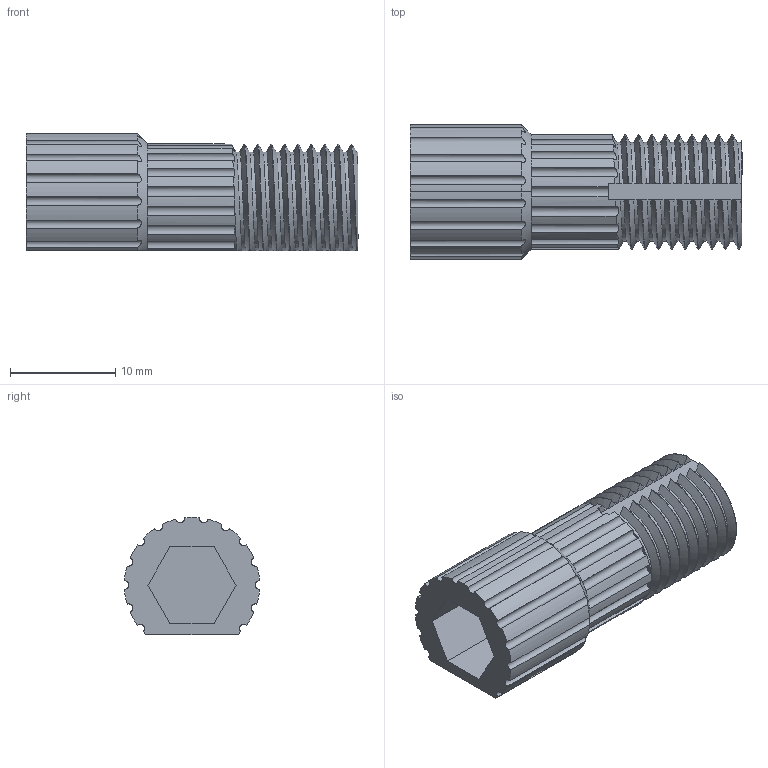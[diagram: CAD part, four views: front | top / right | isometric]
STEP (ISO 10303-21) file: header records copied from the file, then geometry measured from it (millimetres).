
FILE_DESCRIPTION (( 'STEP AP203' ), '1' );
FILE_NAME ('AF-HF-LR-PRT-003-STEP.STEP', '2020-10-04T16:07:10', ( '' ), ( '' ), 'SwSTEP 2.0', 'SolidWorks 2018', '' );
FILE_SCHEMA (( 'CONFIG_CONTROL_DESIGN' ));
Products named in the file (1): AF-HF-LR-PRT-003-STEP
Bounding box: 31.5 x 12.81 x 11.12 mm (x, y, z)
Volume: 2442.1 mm3; surface area: 1936.2 mm2
Topology: 1 solids, 1 shells, 232 faces, 599 edges, 371 vertices
Faces by surface type: cylinder 90, plane 81, bspline 59, cone 2
Entity records: 26712 total; most frequent: CARTESIAN_POINT 21714, ORIENTED_EDGE 1198, DIRECTION 841, EDGE_CURVE 599, VERTEX_POINT 371, AXIS2_PLACEMENT_3D 300, VECTOR 241, LINE 241
